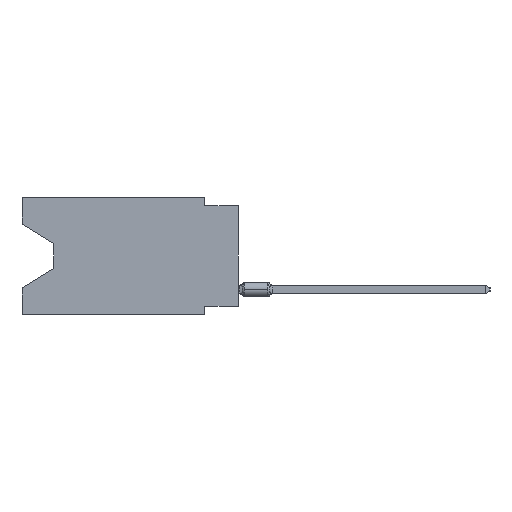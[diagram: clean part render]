
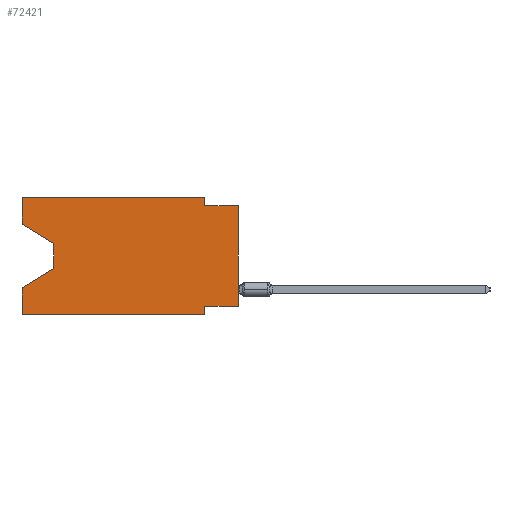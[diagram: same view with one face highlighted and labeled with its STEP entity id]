
A CAD part, left-side view. The second image highlights one B-rep face of the part: STEP entity #72421.
In plain terms, the highlighted planar face has unit normal (-1, 0, 0).
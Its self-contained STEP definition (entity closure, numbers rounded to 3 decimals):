
#998 = CARTESIAN_POINT ( 'NONE',  ( 0., 0., -8.255 ) ) ;
#1670 = VECTOR ( 'NONE', #58292, 1000. ) ;
#3086 = LINE ( 'NONE', #60368, #77766 ) ;
#3957 = CARTESIAN_POINT ( 'NONE',  ( 0., 0., -8.255 ) ) ;
#6070 = EDGE_CURVE ( 'NONE', #26306, #9953, #33290, .T. ) ;
#7151 = VERTEX_POINT ( 'NONE', #25518 ) ;
#7632 = CARTESIAN_POINT ( 'NONE',  ( 0., 2.54, -8.89 ) ) ;
#8016 = CARTESIAN_POINT ( 'NONE',  ( 0., 16.383, -6.852 ) ) ;
#9953 = VERTEX_POINT ( 'NONE', #8016 ) ;
#10278 = VERTEX_POINT ( 'NONE', #54715 ) ;
#10597 = VERTEX_POINT ( 'NONE', #88928 ) ;
#10956 = ORIENTED_EDGE ( 'NONE', *, *, #87372, .F. ) ;
#12162 = LINE ( 'NONE', #40140, #58159 ) ;
#12975 = VECTOR ( 'NONE', #72931, 1000. ) ;
#13993 = CARTESIAN_POINT ( 'NONE',  ( 0., 2.54, -0.635 ) ) ;
#14143 = DIRECTION ( 'NONE',  ( 0., 0., -1. ) ) ;
#14946 = CARTESIAN_POINT ( 'NONE',  ( 0., 2.54, 0. ) ) ;
#15188 = LINE ( 'NONE', #998, #46321 ) ;
#15723 = EDGE_CURVE ( 'NONE', #40555, #10597, #55853, .T. ) ;
#15852 = DIRECTION ( 'NONE',  ( 0., 0., -1. ) ) ;
#19699 = VECTOR ( 'NONE', #87620, 1000. ) ;
#22223 = CARTESIAN_POINT ( 'NONE',  ( 0., 16.383, -8.89 ) ) ;
#23954 = ORIENTED_EDGE ( 'NONE', *, *, #25099, .T. ) ;
#23958 = DIRECTION ( 'NONE',  ( 1., 0., 0. ) ) ;
#24336 = CARTESIAN_POINT ( 'NONE',  ( 0., 16.383, 0. ) ) ;
#25099 = EDGE_CURVE ( 'NONE', #64278, #32158, #12162, .T. ) ;
#25518 = CARTESIAN_POINT ( 'NONE',  ( 0., 2.54, -8.255 ) ) ;
#26098 = VERTEX_POINT ( 'NONE', #65833 ) ;
#26306 = VERTEX_POINT ( 'NONE', #76336 ) ;
#30868 = FACE_OUTER_BOUND ( 'NONE', #41878, .T. ) ;
#30915 = LINE ( 'NONE', #52443, #31933 ) ;
#31933 = VECTOR ( 'NONE', #72602, 1000. ) ;
#32158 = VERTEX_POINT ( 'NONE', #89897 ) ;
#32839 = DIRECTION ( 'NONE',  ( 0., 0.855, -0.519 ) ) ;
#33290 = LINE ( 'NONE', #74536, #73122 ) ;
#36623 = VECTOR ( 'NONE', #14143, 1000. ) ;
#36873 = CARTESIAN_POINT ( 'NONE',  ( 0., 16.383, -2.038 ) ) ;
#40140 = CARTESIAN_POINT ( 'NONE',  ( 0., 16.383, -2.038 ) ) ;
#40555 = VERTEX_POINT ( 'NONE', #13993 ) ;
#41316 = DIRECTION ( 'NONE',  ( 0., -1., 0. ) ) ;
#41878 = EDGE_LOOP ( 'NONE', ( #23954, #54523, #49955, #63649, #54205, #57934, #57250, #84839, #73222, #50941, #10956, #55212 ) ) ;
#42096 = DIRECTION ( 'NONE',  ( 0., -1., 0. ) ) ;
#43654 = LINE ( 'NONE', #51431, #12975 ) ;
#46175 = DIRECTION ( 'NONE',  ( 0., 0., 1. ) ) ;
#46321 = VECTOR ( 'NONE', #83933, 1000. ) ;
#48058 = CARTESIAN_POINT ( 'NONE',  ( 0., 16.383, -8.89 ) ) ;
#48447 = EDGE_CURVE ( 'NONE', #81525, #10597, #43654, .T. ) ;
#49125 = VERTEX_POINT ( 'NONE', #48058 ) ;
#49874 = CARTESIAN_POINT ( 'NONE',  ( 0., 0., -0.635 ) ) ;
#49955 = ORIENTED_EDGE ( 'NONE', *, *, #6070, .T. ) ;
#50941 = ORIENTED_EDGE ( 'NONE', *, *, #53808, .F. ) ;
#51431 = CARTESIAN_POINT ( 'NONE',  ( 0., 0., 0. ) ) ;
#52443 = CARTESIAN_POINT ( 'NONE',  ( 0., 13.97, -3.505 ) ) ;
#52761 = LINE ( 'NONE', #24336, #1670 ) ;
#53569 = EDGE_CURVE ( 'NONE', #64278, #10278, #3086, .T. ) ;
#53808 = EDGE_CURVE ( 'NONE', #26098, #40555, #72198, .T. ) ;
#54205 = ORIENTED_EDGE ( 'NONE', *, *, #61950, .T. ) ;
#54523 = ORIENTED_EDGE ( 'NONE', *, *, #84047, .T. ) ;
#54715 = CARTESIAN_POINT ( 'NONE',  ( 0., 16.383, 0. ) ) ;
#55212 = ORIENTED_EDGE ( 'NONE', *, *, #53569, .F. ) ;
#55853 = LINE ( 'NONE', #49874, #85860 ) ;
#57250 = ORIENTED_EDGE ( 'NONE', *, *, #66705, .F. ) ;
#57315 = VECTOR ( 'NONE', #41316, 1000. ) ;
#57934 = ORIENTED_EDGE ( 'NONE', *, *, #60494, .F. ) ;
#58159 = VECTOR ( 'NONE', #68982, 1000. ) ;
#58292 = DIRECTION ( 'NONE',  ( 0., -1., 0. ) ) ;
#58436 = LINE ( 'NONE', #22223, #57315 ) ;
#58821 = PLANE ( 'NONE',  #88219 ) ;
#59271 = DIRECTION ( 'NONE',  ( 0., 0., -1. ) ) ;
#60368 = CARTESIAN_POINT ( 'NONE',  ( 0., 16.383, 0. ) ) ;
#60494 = EDGE_CURVE ( 'NONE', #7151, #64670, #64091, .T. ) ;
#61497 = CARTESIAN_POINT ( 'NONE',  ( 0., 2.54, -8.89 ) ) ;
#61950 = EDGE_CURVE ( 'NONE', #49125, #64670, #58436, .T. ) ;
#63649 = ORIENTED_EDGE ( 'NONE', *, *, #80206, .F. ) ;
#64091 = LINE ( 'NONE', #61497, #36623 ) ;
#64278 = VERTEX_POINT ( 'NONE', #36873 ) ;
#64670 = VERTEX_POINT ( 'NONE', #7632 ) ;
#65833 = CARTESIAN_POINT ( 'NONE',  ( 0., 2.54, 0. ) ) ;
#66705 = EDGE_CURVE ( 'NONE', #81525, #7151, #15188, .T. ) ;
#68982 = DIRECTION ( 'NONE',  ( 0., -0.855, -0.519 ) ) ;
#72198 = LINE ( 'NONE', #14946, #86482 ) ;
#72421 = ADVANCED_FACE ( 'NONE', ( #30868 ), #58821, .F. ) ;
#72602 = DIRECTION ( 'NONE',  ( 0., 0., -1. ) ) ;
#72931 = DIRECTION ( 'NONE',  ( 0., 0., 1. ) ) ;
#73122 = VECTOR ( 'NONE', #32839, 1000. ) ;
#73222 = ORIENTED_EDGE ( 'NONE', *, *, #15723, .F. ) ;
#74536 = CARTESIAN_POINT ( 'NONE',  ( 0., 13.97, -5.385 ) ) ;
#76336 = CARTESIAN_POINT ( 'NONE',  ( 0., 13.97, -5.385 ) ) ;
#77766 = VECTOR ( 'NONE', #46175, 1000. ) ;
#80206 = EDGE_CURVE ( 'NONE', #49125, #9953, #88072, .T. ) ;
#81525 = VERTEX_POINT ( 'NONE', #3957 ) ;
#83933 = DIRECTION ( 'NONE',  ( 0., 1., 0. ) ) ;
#84047 = EDGE_CURVE ( 'NONE', #32158, #26306, #30915, .T. ) ;
#84839 = ORIENTED_EDGE ( 'NONE', *, *, #48447, .T. ) ;
#85860 = VECTOR ( 'NONE', #42096, 1000. ) ;
#86482 = VECTOR ( 'NONE', #15852, 1000. ) ;
#86718 = CARTESIAN_POINT ( 'NONE',  ( 0., 16.383, 0. ) ) ;
#87171 = CARTESIAN_POINT ( 'NONE',  ( 0., 16.383, 0. ) ) ;
#87372 = EDGE_CURVE ( 'NONE', #10278, #26098, #52761, .T. ) ;
#87620 = DIRECTION ( 'NONE',  ( 0., 0., 1. ) ) ;
#88072 = LINE ( 'NONE', #87171, #19699 ) ;
#88219 = AXIS2_PLACEMENT_3D ( 'NONE', #86718, #23958, #59271 ) ;
#88928 = CARTESIAN_POINT ( 'NONE',  ( 0., 0., -0.635 ) ) ;
#89897 = CARTESIAN_POINT ( 'NONE',  ( 0., 13.97, -3.505 ) ) ;
